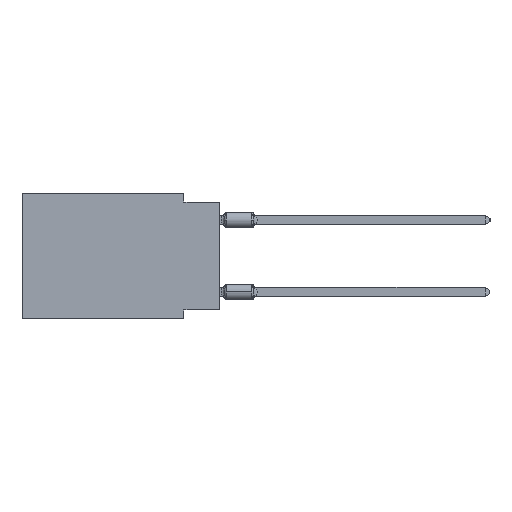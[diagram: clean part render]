
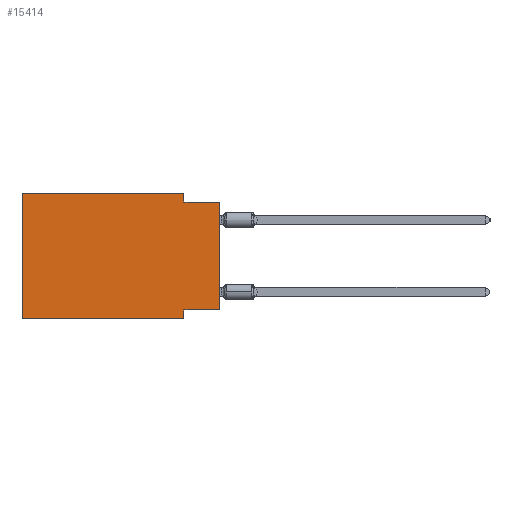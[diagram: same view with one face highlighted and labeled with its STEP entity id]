
A CAD part, left-side view. The second image highlights one B-rep face of the part: STEP entity #15414.
In plain terms, the highlighted planar face has unit normal (-1, 0, 0).
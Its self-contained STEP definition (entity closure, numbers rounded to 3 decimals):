
#982 = DIRECTION ( 'NONE',  ( 0., 0., -1. ) ) ;
#2504 = VERTEX_POINT ( 'NONE', #23266 ) ;
#4311 = VERTEX_POINT ( 'NONE', #19277 ) ;
#4607 = LINE ( 'NONE', #6199, #41666 ) ;
#5575 = ORIENTED_EDGE ( 'NONE', *, *, #44177, .F. ) ;
#6199 = CARTESIAN_POINT ( 'NONE',  ( 0., 2.54, -8.89 ) ) ;
#6435 = DIRECTION ( 'NONE',  ( 0., 0., 1. ) ) ;
#6593 = VERTEX_POINT ( 'NONE', #30517 ) ;
#7015 = EDGE_CURVE ( 'NONE', #37688, #21482, #50146, .T. ) ;
#9243 = LINE ( 'NONE', #9764, #26634 ) ;
#9764 = CARTESIAN_POINT ( 'NONE',  ( 0., 0., -8.255 ) ) ;
#10216 = LINE ( 'NONE', #25313, #26739 ) ;
#10473 = ORIENTED_EDGE ( 'NONE', *, *, #38817, .T. ) ;
#10479 = AXIS2_PLACEMENT_3D ( 'NONE', #36773, #36012, #982 ) ;
#10541 = VERTEX_POINT ( 'NONE', #21527 ) ;
#12803 = VECTOR ( 'NONE', #6435, 1000. ) ;
#13088 = CARTESIAN_POINT ( 'NONE',  ( 0., 13.97, 0. ) ) ;
#13398 = EDGE_CURVE ( 'NONE', #4311, #17893, #49056, .T. ) ;
#13449 = LINE ( 'NONE', #44625, #38089 ) ;
#13780 = DIRECTION ( 'NONE',  ( 0., -1., 0. ) ) ;
#14884 = VECTOR ( 'NONE', #13780, 1000. ) ;
#15414 = ADVANCED_FACE ( 'NONE', ( #40863 ), #43948, .F. ) ;
#17893 = VERTEX_POINT ( 'NONE', #38558 ) ;
#18140 = DIRECTION ( 'NONE',  ( 0., 0., -1. ) ) ;
#19173 = ORIENTED_EDGE ( 'NONE', *, *, #45583, .F. ) ;
#19277 = CARTESIAN_POINT ( 'NONE',  ( 0., 13.97, 0. ) ) ;
#21364 = CARTESIAN_POINT ( 'NONE',  ( 0., 0., -8.255 ) ) ;
#21482 = VERTEX_POINT ( 'NONE', #28488 ) ;
#21525 = LINE ( 'NONE', #13088, #45313 ) ;
#21527 = CARTESIAN_POINT ( 'NONE',  ( 0., 13.97, -8.89 ) ) ;
#23266 = CARTESIAN_POINT ( 'NONE',  ( 0., 2.54, -0.635 ) ) ;
#23828 = ORIENTED_EDGE ( 'NONE', *, *, #37334, .F. ) ;
#24600 = DIRECTION ( 'NONE',  ( 0., 1., 0. ) ) ;
#24691 = DIRECTION ( 'NONE',  ( 0., -1., 0. ) ) ;
#25313 = CARTESIAN_POINT ( 'NONE',  ( 0., 2.54, 0. ) ) ;
#25621 = ORIENTED_EDGE ( 'NONE', *, *, #32111, .F. ) ;
#26435 = EDGE_LOOP ( 'NONE', ( #42296, #33108, #19173, #34382, #23828, #10473, #25621, #5575 ) ) ;
#26634 = VECTOR ( 'NONE', #24600, 1000. ) ;
#26739 = VECTOR ( 'NONE', #18140, 1000. ) ;
#28488 = CARTESIAN_POINT ( 'NONE',  ( 0., 0., -0.635 ) ) ;
#30517 = CARTESIAN_POINT ( 'NONE',  ( 0., 2.54, -8.255 ) ) ;
#32111 = EDGE_CURVE ( 'NONE', #6593, #44134, #4607, .T. ) ;
#32264 = CARTESIAN_POINT ( 'NONE',  ( 0., 2.54, -8.89 ) ) ;
#33108 = ORIENTED_EDGE ( 'NONE', *, *, #47698, .F. ) ;
#33109 = LINE ( 'NONE', #36684, #50416 ) ;
#34382 = ORIENTED_EDGE ( 'NONE', *, *, #13398, .F. ) ;
#36012 = DIRECTION ( 'NONE',  ( 1., 0., 0. ) ) ;
#36684 = CARTESIAN_POINT ( 'NONE',  ( 0., 0., -0.635 ) ) ;
#36773 = CARTESIAN_POINT ( 'NONE',  ( 0., 13.97, 0. ) ) ;
#37334 = EDGE_CURVE ( 'NONE', #10541, #4311, #21525, .T. ) ;
#37688 = VERTEX_POINT ( 'NONE', #21364 ) ;
#38089 = VECTOR ( 'NONE', #24691, 1000. ) ;
#38558 = CARTESIAN_POINT ( 'NONE',  ( 0., 2.54, 0. ) ) ;
#38817 = EDGE_CURVE ( 'NONE', #10541, #44134, #13449, .T. ) ;
#40860 = CARTESIAN_POINT ( 'NONE',  ( 0., 13.97, 0. ) ) ;
#40863 = FACE_OUTER_BOUND ( 'NONE', #26435, .T. ) ;
#41446 = CARTESIAN_POINT ( 'NONE',  ( 0., 0., 0. ) ) ;
#41666 = VECTOR ( 'NONE', #42699, 1000. ) ;
#42296 = ORIENTED_EDGE ( 'NONE', *, *, #7015, .T. ) ;
#42699 = DIRECTION ( 'NONE',  ( 0., 0., -1. ) ) ;
#43948 = PLANE ( 'NONE',  #10479 ) ;
#44134 = VERTEX_POINT ( 'NONE', #32264 ) ;
#44177 = EDGE_CURVE ( 'NONE', #37688, #6593, #9243, .T. ) ;
#44625 = CARTESIAN_POINT ( 'NONE',  ( 0., 13.97, -8.89 ) ) ;
#45313 = VECTOR ( 'NONE', #47598, 1000. ) ;
#45583 = EDGE_CURVE ( 'NONE', #17893, #2504, #10216, .T. ) ;
#47598 = DIRECTION ( 'NONE',  ( 0., 0., 1. ) ) ;
#47698 = EDGE_CURVE ( 'NONE', #2504, #21482, #33109, .T. ) ;
#48724 = DIRECTION ( 'NONE',  ( 0., -1., 0. ) ) ;
#49056 = LINE ( 'NONE', #40860, #14884 ) ;
#50146 = LINE ( 'NONE', #41446, #12803 ) ;
#50416 = VECTOR ( 'NONE', #48724, 1000. ) ;
